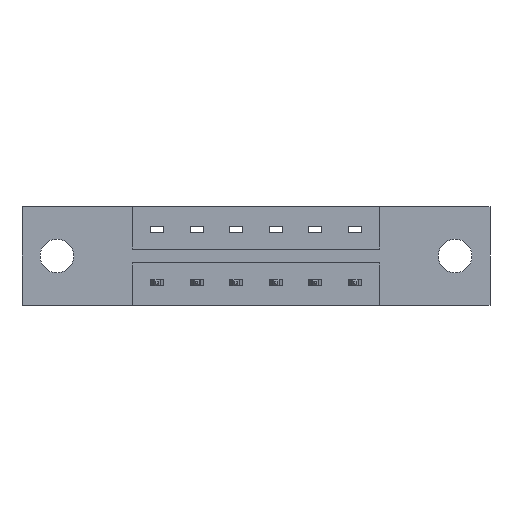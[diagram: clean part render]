
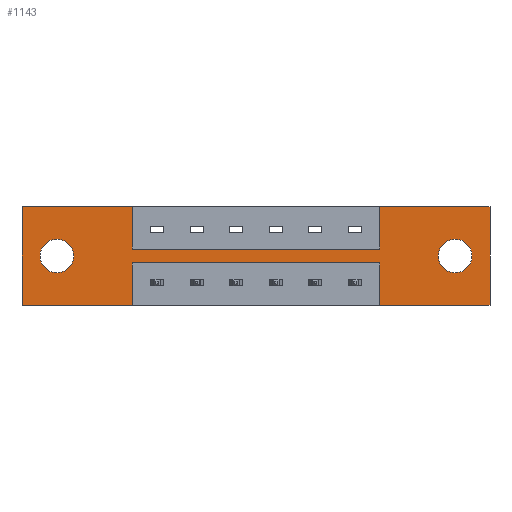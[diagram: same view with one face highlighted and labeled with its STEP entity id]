
A CAD part, front view. The second image highlights one B-rep face of the part: STEP entity #1143.
In plain terms, the highlighted planar face has unit normal (0, -1, 0).
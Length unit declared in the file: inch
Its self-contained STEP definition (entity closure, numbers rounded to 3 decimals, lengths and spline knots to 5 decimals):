
#70 = EDGE_CURVE ( 'NONE', #479, #5825, #188, .T. ) ;
#130 = EDGE_LOOP ( 'NONE', ( #5655, #3118 ) ) ;
#188 = LINE ( 'NONE', #2822, #6322 ) ;
#189 = VERTEX_POINT ( 'NONE', #6868 ) ;
#257 = CIRCLE ( 'NONE', #8300, 0.064 ) ;
#305 = EDGE_CURVE ( 'NONE', #4986, #3053, #6924, .T. ) ;
#316 = DIRECTION ( 'NONE',  ( 1., 0., 0. ) ) ;
#370 = ORIENTED_EDGE ( 'NONE', *, *, #4541, .F. ) ;
#375 = CARTESIAN_POINT ( 'NONE',  ( 1.3575, 0., -0.214 ) ) ;
#464 = EDGE_CURVE ( 'NONE', #3799, #4918, #1060, .T. ) ;
#473 = CARTESIAN_POINT ( 'NONE',  ( 1.3575, 0., -0.214 ) ) ;
#479 = VERTEX_POINT ( 'NONE', #473 ) ;
#481 = ORIENTED_EDGE ( 'NONE', *, *, #8043, .T. ) ;
#519 = LINE ( 'NONE', #6161, #1910 ) ;
#537 = LINE ( 'NONE', #7581, #7381 ) ;
#649 = VECTOR ( 'NONE', #2292, 39.37008 ) ;
#743 = CARTESIAN_POINT ( 'NONE',  ( 0.1325, 0., -0.1235 ) ) ;
#822 = CARTESIAN_POINT ( 'NONE',  ( 0.4175, 0., -0.375 ) ) ;
#884 = VERTEX_POINT ( 'NONE', #5219 ) ;
#991 = CARTESIAN_POINT ( 'NONE',  ( 1.6425, 0., -0.1875 ) ) ;
#1060 = CIRCLE ( 'NONE', #7505, 0.064 ) ;
#1143 = ADVANCED_FACE ( 'NONE', ( #2850, #6502, #2151 ), #1519, .T. ) ;
#1215 = LINE ( 'NONE', #7501, #7887 ) ;
#1292 = VERTEX_POINT ( 'NONE', #2910 ) ;
#1384 = DIRECTION ( 'NONE',  ( 0., 0., -1. ) ) ;
#1519 = PLANE ( 'NONE',  #6557 ) ;
#1685 = ORIENTED_EDGE ( 'NONE', *, *, #5168, .F. ) ;
#1803 = DIRECTION ( 'NONE',  ( 0., 0., 1. ) ) ;
#1838 = DIRECTION ( 'NONE',  ( -1., 0., 0. ) ) ;
#1901 = LINE ( 'NONE', #1993, #2502 ) ;
#1910 = VECTOR ( 'NONE', #4276, 39.37008 ) ;
#1914 = CARTESIAN_POINT ( 'NONE',  ( 0., 0., -0.375 ) ) ;
#1993 = CARTESIAN_POINT ( 'NONE',  ( 0.4175, 0., -0.214 ) ) ;
#1997 = EDGE_CURVE ( 'NONE', #4971, #2233, #5264, .T. ) ;
#2025 = VECTOR ( 'NONE', #5161, 39.37008 ) ;
#2139 = CARTESIAN_POINT ( 'NONE',  ( 0., 0., -0.375 ) ) ;
#2151 = FACE_OUTER_BOUND ( 'NONE', #3172, .T. ) ;
#2153 = AXIS2_PLACEMENT_3D ( 'NONE', #991, #7387, #6074 ) ;
#2228 = CARTESIAN_POINT ( 'NONE',  ( 0.4175, 0., -0.214 ) ) ;
#2233 = VERTEX_POINT ( 'NONE', #2139 ) ;
#2292 = DIRECTION ( 'NONE',  ( 0., 0., 1. ) ) ;
#2323 = EDGE_CURVE ( 'NONE', #4604, #1292, #519, .T. ) ;
#2357 = DIRECTION ( 'NONE',  ( 0., 1., 0. ) ) ;
#2443 = ORIENTED_EDGE ( 'NONE', *, *, #2650, .F. ) ;
#2492 = DIRECTION ( 'NONE',  ( 0., 0., -1. ) ) ;
#2502 = VECTOR ( 'NONE', #1384, 39.37008 ) ;
#2650 = EDGE_CURVE ( 'NONE', #5825, #4971, #1901, .T. ) ;
#2822 = CARTESIAN_POINT ( 'NONE',  ( 0.4175, 0., -0.214 ) ) ;
#2825 = CARTESIAN_POINT ( 'NONE',  ( 1.3575, 0., -0.161 ) ) ;
#2850 = FACE_BOUND ( 'NONE', #3045, .T. ) ;
#2881 = VECTOR ( 'NONE', #4051, 39.37008 ) ;
#2895 = CARTESIAN_POINT ( 'NONE',  ( 0., 0., 0. ) ) ;
#2910 = CARTESIAN_POINT ( 'NONE',  ( 0.4175, 0., 0. ) ) ;
#2942 = LINE ( 'NONE', #6174, #649 ) ;
#3045 = EDGE_LOOP ( 'NONE', ( #6238, #481 ) ) ;
#3053 = VERTEX_POINT ( 'NONE', #8263 ) ;
#3118 = ORIENTED_EDGE ( 'NONE', *, *, #464, .T. ) ;
#3172 = EDGE_LOOP ( 'NONE', ( #1685, #5334, #3291, #370, #5038, #3791, #3783, #3934, #4611, #3333, #2443, #7628 ) ) ;
#3291 = ORIENTED_EDGE ( 'NONE', *, *, #5573, .F. ) ;
#3293 = CARTESIAN_POINT ( 'NONE',  ( 1.775, 0., 0. ) ) ;
#3333 = ORIENTED_EDGE ( 'NONE', *, *, #1997, .F. ) ;
#3444 = VERTEX_POINT ( 'NONE', #2825 ) ;
#3457 = EDGE_CURVE ( 'NONE', #4918, #3799, #4614, .T. ) ;
#3491 = CARTESIAN_POINT ( 'NONE',  ( 0., 0., 0. ) ) ;
#3636 = DIRECTION ( 'NONE',  ( 1., 0., 0. ) ) ;
#3783 = ORIENTED_EDGE ( 'NONE', *, *, #4808, .F. ) ;
#3791 = ORIENTED_EDGE ( 'NONE', *, *, #5886, .F. ) ;
#3799 = VERTEX_POINT ( 'NONE', #7800 ) ;
#3934 = ORIENTED_EDGE ( 'NONE', *, *, #2323, .F. ) ;
#3959 = DIRECTION ( 'NONE',  ( 0., 0., -1. ) ) ;
#4051 = DIRECTION ( 'NONE',  ( 0., 0., 1. ) ) ;
#4075 = CARTESIAN_POINT ( 'NONE',  ( 1.3575, 0., -0.161 ) ) ;
#4108 = DIRECTION ( 'NONE',  ( -1., 0., 0. ) ) ;
#4122 = DIRECTION ( 'NONE',  ( 0., -1., 0. ) ) ;
#4221 = VERTEX_POINT ( 'NONE', #7639 ) ;
#4276 = DIRECTION ( 'NONE',  ( 1., 0., 0. ) ) ;
#4522 = EDGE_CURVE ( 'NONE', #3444, #4221, #4599, .T. ) ;
#4541 = EDGE_CURVE ( 'NONE', #4221, #4755, #7626, .T. ) ;
#4599 = LINE ( 'NONE', #4075, #2881 ) ;
#4604 = VERTEX_POINT ( 'NONE', #2895 ) ;
#4611 = ORIENTED_EDGE ( 'NONE', *, *, #8055, .F. ) ;
#4614 = CIRCLE ( 'NONE', #5133, 0.064 ) ;
#4755 = VERTEX_POINT ( 'NONE', #6944 ) ;
#4783 = CARTESIAN_POINT ( 'NONE',  ( 1.3575, 0., -0.375 ) ) ;
#4808 = EDGE_CURVE ( 'NONE', #1292, #884, #537, .T. ) ;
#4918 = VERTEX_POINT ( 'NONE', #743 ) ;
#4971 = VERTEX_POINT ( 'NONE', #822 ) ;
#4986 = VERTEX_POINT ( 'NONE', #6040 ) ;
#5038 = ORIENTED_EDGE ( 'NONE', *, *, #4522, .F. ) ;
#5133 = AXIS2_PLACEMENT_3D ( 'NONE', #7975, #6761, #7345 ) ;
#5161 = DIRECTION ( 'NONE',  ( -1., 0., 0. ) ) ;
#5168 = EDGE_CURVE ( 'NONE', #7572, #479, #5776, .T. ) ;
#5219 = CARTESIAN_POINT ( 'NONE',  ( 0.4175, 0., -0.161 ) ) ;
#5264 = LINE ( 'NONE', #1914, #6776 ) ;
#5276 = LINE ( 'NONE', #3293, #7087 ) ;
#5334 = ORIENTED_EDGE ( 'NONE', *, *, #5585, .F. ) ;
#5389 = LINE ( 'NONE', #7720, #2025 ) ;
#5573 = EDGE_CURVE ( 'NONE', #4755, #189, #5276, .T. ) ;
#5585 = EDGE_CURVE ( 'NONE', #189, #7572, #5389, .T. ) ;
#5655 = ORIENTED_EDGE ( 'NONE', *, *, #3457, .T. ) ;
#5776 = LINE ( 'NONE', #375, #7678 ) ;
#5825 = VERTEX_POINT ( 'NONE', #2228 ) ;
#5886 = EDGE_CURVE ( 'NONE', #884, #3444, #1215, .T. ) ;
#5922 = VECTOR ( 'NONE', #316, 39.37008 ) ;
#6040 = CARTESIAN_POINT ( 'NONE',  ( 1.6425, 0., -0.1235 ) ) ;
#6069 = CARTESIAN_POINT ( 'NONE',  ( 0., 0., -0.375 ) ) ;
#6074 = DIRECTION ( 'NONE',  ( 0., 0., -1. ) ) ;
#6148 = DIRECTION ( 'NONE',  ( 0., 0., -1. ) ) ;
#6161 = CARTESIAN_POINT ( 'NONE',  ( 0., 0., 0. ) ) ;
#6174 = CARTESIAN_POINT ( 'NONE',  ( 0., 0., 0. ) ) ;
#6238 = ORIENTED_EDGE ( 'NONE', *, *, #305, .T. ) ;
#6245 = CARTESIAN_POINT ( 'NONE',  ( 0.1325, 0., -0.1875 ) ) ;
#6322 = VECTOR ( 'NONE', #4108, 39.37008 ) ;
#6502 = FACE_BOUND ( 'NONE', #130, .T. ) ;
#6557 = AXIS2_PLACEMENT_3D ( 'NONE', #6069, #4122, #7382 ) ;
#6672 = DIRECTION ( 'NONE',  ( 0., 0., 1. ) ) ;
#6761 = DIRECTION ( 'NONE',  ( 0., 1., 0. ) ) ;
#6776 = VECTOR ( 'NONE', #1838, 39.37008 ) ;
#6868 = CARTESIAN_POINT ( 'NONE',  ( 1.775, 0., -0.375 ) ) ;
#6924 = CIRCLE ( 'NONE', #2153, 0.064 ) ;
#6944 = CARTESIAN_POINT ( 'NONE',  ( 1.775, 0., 0. ) ) ;
#7087 = VECTOR ( 'NONE', #3959, 39.37008 ) ;
#7345 = DIRECTION ( 'NONE',  ( 0., 0., 1. ) ) ;
#7381 = VECTOR ( 'NONE', #2492, 39.37008 ) ;
#7382 = DIRECTION ( 'NONE',  ( 0., 0., -1. ) ) ;
#7387 = DIRECTION ( 'NONE',  ( 0., 1., 0. ) ) ;
#7501 = CARTESIAN_POINT ( 'NONE',  ( 0.4175, 0., -0.161 ) ) ;
#7505 = AXIS2_PLACEMENT_3D ( 'NONE', #6245, #2357, #1803 ) ;
#7572 = VERTEX_POINT ( 'NONE', #4783 ) ;
#7581 = CARTESIAN_POINT ( 'NONE',  ( 0.4175, 0., -0.161 ) ) ;
#7626 = LINE ( 'NONE', #3491, #5922 ) ;
#7628 = ORIENTED_EDGE ( 'NONE', *, *, #70, .F. ) ;
#7639 = CARTESIAN_POINT ( 'NONE',  ( 1.3575, 0., 0. ) ) ;
#7678 = VECTOR ( 'NONE', #6672, 39.37008 ) ;
#7720 = CARTESIAN_POINT ( 'NONE',  ( 0., 0., -0.375 ) ) ;
#7800 = CARTESIAN_POINT ( 'NONE',  ( 0.1325, 0., -0.2515 ) ) ;
#7883 = DIRECTION ( 'NONE',  ( 0., 1., 0. ) ) ;
#7887 = VECTOR ( 'NONE', #3636, 39.37008 ) ;
#7975 = CARTESIAN_POINT ( 'NONE',  ( 0.1325, 0., -0.1875 ) ) ;
#8043 = EDGE_CURVE ( 'NONE', #3053, #4986, #257, .T. ) ;
#8055 = EDGE_CURVE ( 'NONE', #2233, #4604, #2942, .T. ) ;
#8061 = CARTESIAN_POINT ( 'NONE',  ( 1.6425, 0., -0.1875 ) ) ;
#8263 = CARTESIAN_POINT ( 'NONE',  ( 1.6425, 0., -0.2515 ) ) ;
#8300 = AXIS2_PLACEMENT_3D ( 'NONE', #8061, #7883, #6148 ) ;
